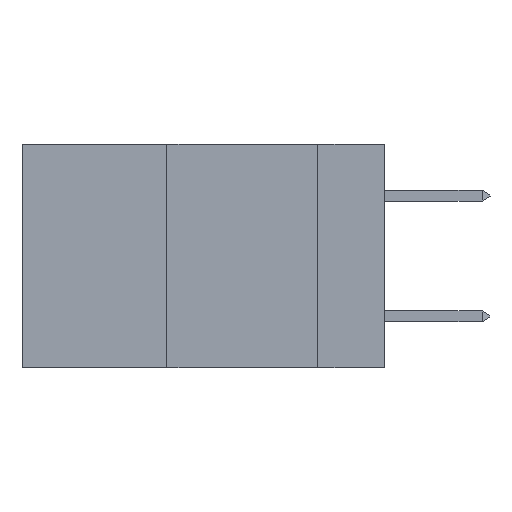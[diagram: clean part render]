
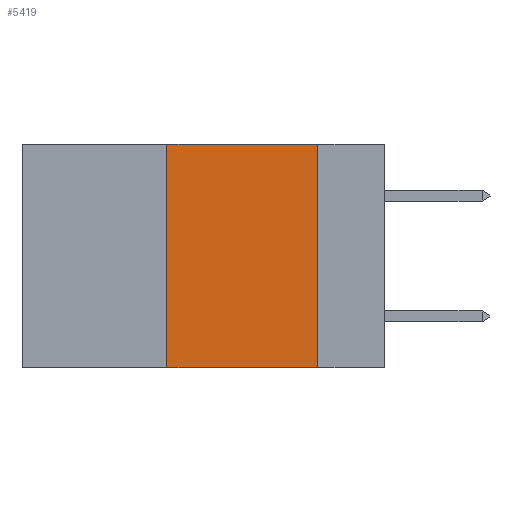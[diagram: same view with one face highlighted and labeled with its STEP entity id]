
A CAD part, left-side view. The second image highlights one B-rep face of the part: STEP entity #5419.
In plain terms, the highlighted planar face has unit normal (-1, 0, 0).
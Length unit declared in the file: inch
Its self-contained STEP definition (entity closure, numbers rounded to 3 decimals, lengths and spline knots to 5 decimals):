
#515 = DIRECTION ( 'NONE',  ( 0., -1., 0. ) ) ;
#1663 = DIRECTION ( 'NONE',  ( 0., 0., 1. ) ) ;
#3297 = LINE ( 'NONE', #29119, #26513 ) ;
#3560 = CARTESIAN_POINT ( 'NONE',  ( 0., 0.36, 0. ) ) ;
#4292 = FACE_OUTER_BOUND ( 'NONE', #14570, .T. ) ;
#5184 = CARTESIAN_POINT ( 'NONE',  ( 0., 0.11, 0. ) ) ;
#5419 = ADVANCED_FACE ( 'NONE', ( #4292 ), #30998, .F. ) ;
#7243 = EDGE_CURVE ( 'NONE', #12399, #26839, #3297, .T. ) ;
#7245 = DIRECTION ( 'NONE',  ( 0., 0., -1. ) ) ;
#7980 = ORIENTED_EDGE ( 'NONE', *, *, #28800, .F. ) ;
#10384 = AXIS2_PLACEMENT_3D ( 'NONE', #20202, #12769, #7245 ) ;
#12202 = DIRECTION ( 'NONE',  ( 0., -1., 0. ) ) ;
#12399 = VERTEX_POINT ( 'NONE', #3560 ) ;
#12769 = DIRECTION ( 'NONE',  ( 1., 0., 0. ) ) ;
#14570 = EDGE_LOOP ( 'NONE', ( #7980, #29373, #30917, #30306 ) ) ;
#16215 = VERTEX_POINT ( 'NONE', #17129 ) ;
#17129 = CARTESIAN_POINT ( 'NONE',  ( 0., 0.36, -0.37 ) ) ;
#17779 = VECTOR ( 'NONE', #1663, 39.37008 ) ;
#20202 = CARTESIAN_POINT ( 'NONE',  ( 0., 0.6, 0. ) ) ;
#22430 = CARTESIAN_POINT ( 'NONE',  ( 0., 0.6, -0.37 ) ) ;
#22990 = LINE ( 'NONE', #30466, #17779 ) ;
#23128 = LINE ( 'NONE', #22430, #32225 ) ;
#23481 = VECTOR ( 'NONE', #31683, 39.37008 ) ;
#25357 = CARTESIAN_POINT ( 'NONE',  ( 0., 0.11, -0.37 ) ) ;
#26513 = VECTOR ( 'NONE', #515, 39.37008 ) ;
#26839 = VERTEX_POINT ( 'NONE', #5184 ) ;
#27363 = EDGE_CURVE ( 'NONE', #16215, #12399, #22990, .T. ) ;
#27910 = EDGE_CURVE ( 'NONE', #16215, #31438, #23128, .T. ) ;
#28800 = EDGE_CURVE ( 'NONE', #26839, #31438, #29218, .T. ) ;
#29119 = CARTESIAN_POINT ( 'NONE',  ( 0., 0.6, 0. ) ) ;
#29218 = LINE ( 'NONE', #31333, #23481 ) ;
#29373 = ORIENTED_EDGE ( 'NONE', *, *, #7243, .F. ) ;
#30306 = ORIENTED_EDGE ( 'NONE', *, *, #27910, .T. ) ;
#30466 = CARTESIAN_POINT ( 'NONE',  ( 0., 0.36, 0. ) ) ;
#30917 = ORIENTED_EDGE ( 'NONE', *, *, #27363, .F. ) ;
#30998 = PLANE ( 'NONE',  #10384 ) ;
#31333 = CARTESIAN_POINT ( 'NONE',  ( 0., 0.11, 0. ) ) ;
#31438 = VERTEX_POINT ( 'NONE', #25357 ) ;
#31683 = DIRECTION ( 'NONE',  ( 0., 0., -1. ) ) ;
#32225 = VECTOR ( 'NONE', #12202, 39.37008 ) ;
